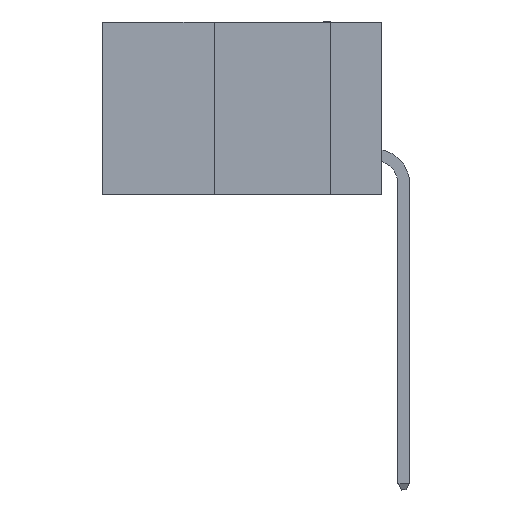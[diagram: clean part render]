
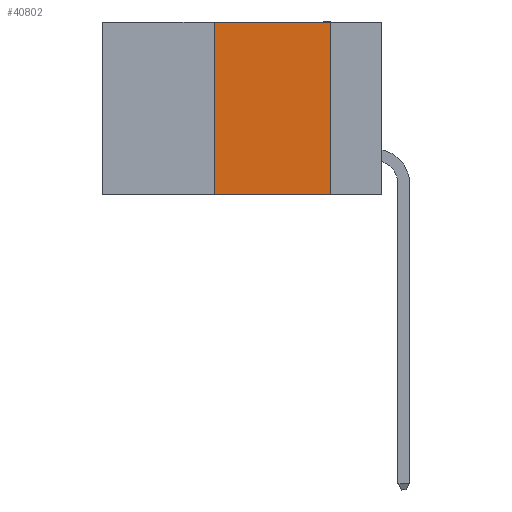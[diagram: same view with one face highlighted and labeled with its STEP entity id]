
A CAD part, left-side view. The second image highlights one B-rep face of the part: STEP entity #40802.
In plain terms, the highlighted planar face has unit normal (-1, 0, 0).
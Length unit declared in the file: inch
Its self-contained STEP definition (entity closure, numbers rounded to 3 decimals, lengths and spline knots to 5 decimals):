
#392 = DIRECTION ( 'NONE',  ( 0., 0., -1. ) ) ;
#1612 = CARTESIAN_POINT ( 'NONE',  ( 0., 0.36, 0. ) ) ;
#2654 = LINE ( 'NONE', #1612, #30894 ) ;
#3098 = LINE ( 'NONE', #5399, #30788 ) ;
#3255 = LINE ( 'NONE', #22069, #15524 ) ;
#3689 = ORIENTED_EDGE ( 'NONE', *, *, #6894, .F. ) ;
#5018 = CARTESIAN_POINT ( 'NONE',  ( 0., 0.11, 0. ) ) ;
#5399 = CARTESIAN_POINT ( 'NONE',  ( 0., 0.6, -0.37 ) ) ;
#5558 = FACE_OUTER_BOUND ( 'NONE', #27288, .T. ) ;
#6476 = ORIENTED_EDGE ( 'NONE', *, *, #18392, .T. ) ;
#6894 = EDGE_CURVE ( 'NONE', #25710, #20945, #2654, .T. ) ;
#9210 = CARTESIAN_POINT ( 'NONE',  ( 0., 0.11, -0.37 ) ) ;
#9575 = VERTEX_POINT ( 'NONE', #9210 ) ;
#15205 = PLANE ( 'NONE',  #33425 ) ;
#15524 = VECTOR ( 'NONE', #42297, 39.37008 ) ;
#16286 = EDGE_CURVE ( 'NONE', #30097, #9575, #18250, .T. ) ;
#17738 = VECTOR ( 'NONE', #392, 39.37008 ) ;
#18008 = CARTESIAN_POINT ( 'NONE',  ( 0., 0.11, 0. ) ) ;
#18250 = LINE ( 'NONE', #18008, #17738 ) ;
#18392 = EDGE_CURVE ( 'NONE', #25710, #9575, #3098, .T. ) ;
#20945 = VERTEX_POINT ( 'NONE', #37137 ) ;
#21607 = DIRECTION ( 'NONE',  ( 0., 0., -1. ) ) ;
#22069 = CARTESIAN_POINT ( 'NONE',  ( 0., 0.6, 0. ) ) ;
#25683 = DIRECTION ( 'NONE',  ( 1., 0., 0. ) ) ;
#25710 = VERTEX_POINT ( 'NONE', #29443 ) ;
#27288 = EDGE_LOOP ( 'NONE', ( #33331, #29307, #3689, #6476 ) ) ;
#28889 = DIRECTION ( 'NONE',  ( 0., 0., 1. ) ) ;
#29307 = ORIENTED_EDGE ( 'NONE', *, *, #33768, .F. ) ;
#29443 = CARTESIAN_POINT ( 'NONE',  ( 0., 0.36, -0.37 ) ) ;
#30097 = VERTEX_POINT ( 'NONE', #5018 ) ;
#30380 = DIRECTION ( 'NONE',  ( 0., -1., 0. ) ) ;
#30788 = VECTOR ( 'NONE', #30380, 39.37008 ) ;
#30894 = VECTOR ( 'NONE', #28889, 39.37008 ) ;
#32039 = CARTESIAN_POINT ( 'NONE',  ( 0., 0.6, 0. ) ) ;
#33331 = ORIENTED_EDGE ( 'NONE', *, *, #16286, .F. ) ;
#33425 = AXIS2_PLACEMENT_3D ( 'NONE', #32039, #25683, #21607 ) ;
#33768 = EDGE_CURVE ( 'NONE', #20945, #30097, #3255, .T. ) ;
#37137 = CARTESIAN_POINT ( 'NONE',  ( 0., 0.36, 0. ) ) ;
#40802 = ADVANCED_FACE ( 'NONE', ( #5558 ), #15205, .F. ) ;
#42297 = DIRECTION ( 'NONE',  ( 0., -1., 0. ) ) ;
